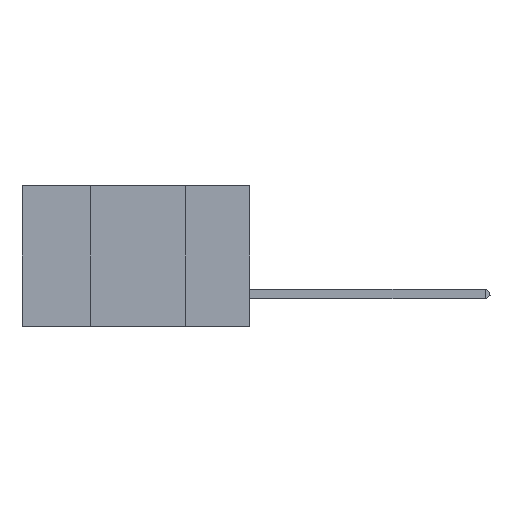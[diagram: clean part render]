
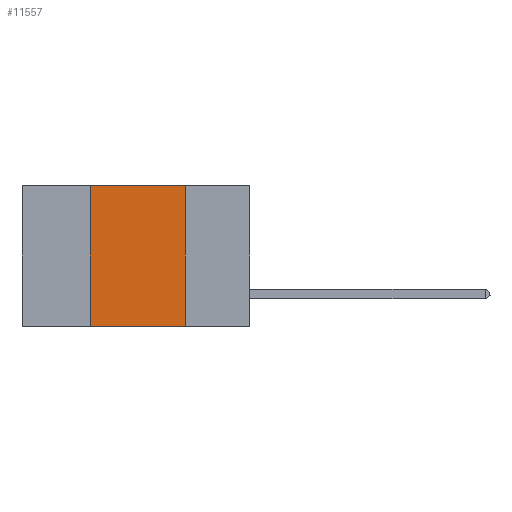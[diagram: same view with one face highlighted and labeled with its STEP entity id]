
A CAD part, left-side view. The second image highlights one B-rep face of the part: STEP entity #11557.
In plain terms, the highlighted planar face has unit normal (-1, 0, 0).
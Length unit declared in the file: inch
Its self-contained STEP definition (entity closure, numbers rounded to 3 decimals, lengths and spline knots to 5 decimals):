
#317 = VECTOR ( 'NONE', #8562, 39.37008 ) ;
#1373 = ORIENTED_EDGE ( 'NONE', *, *, #22876, .F. ) ;
#2792 = CARTESIAN_POINT ( 'NONE',  ( 0., 0.17, 0. ) ) ;
#3092 = PLANE ( 'NONE',  #29829 ) ;
#4129 = ORIENTED_EDGE ( 'NONE', *, *, #28291, .F. ) ;
#4709 = ORIENTED_EDGE ( 'NONE', *, *, #6818, .F. ) ;
#4942 = CARTESIAN_POINT ( 'NONE',  ( 0., 0.6, 0. ) ) ;
#5448 = DIRECTION ( 'NONE',  ( 0., -1., 0. ) ) ;
#5507 = VECTOR ( 'NONE', #21435, 39.37008 ) ;
#6730 = CARTESIAN_POINT ( 'NONE',  ( 0., 0.42, 0. ) ) ;
#6818 = EDGE_CURVE ( 'NONE', #15414, #7684, #13244, .T. ) ;
#7325 = EDGE_LOOP ( 'NONE', ( #1373, #4129, #4709, #10598 ) ) ;
#7684 = VERTEX_POINT ( 'NONE', #6730 ) ;
#7701 = VERTEX_POINT ( 'NONE', #27903 ) ;
#8562 = DIRECTION ( 'NONE',  ( 0., 0., 1. ) ) ;
#10029 = LINE ( 'NONE', #24080, #16336 ) ;
#10276 = DIRECTION ( 'NONE',  ( 0., -1., 0. ) ) ;
#10598 = ORIENTED_EDGE ( 'NONE', *, *, #15586, .T. ) ;
#10708 = CARTESIAN_POINT ( 'NONE',  ( 0., 0.42, 0. ) ) ;
#11557 = ADVANCED_FACE ( 'NONE', ( #23799 ), #3092, .F. ) ;
#13244 = LINE ( 'NONE', #10708, #317 ) ;
#15414 = VERTEX_POINT ( 'NONE', #24898 ) ;
#15586 = EDGE_CURVE ( 'NONE', #15414, #7701, #10029, .T. ) ;
#16336 = VECTOR ( 'NONE', #10276, 39.37008 ) ;
#17015 = DIRECTION ( 'NONE',  ( 1., 0., 0. ) ) ;
#18062 = LINE ( 'NONE', #25851, #5507 ) ;
#19432 = VECTOR ( 'NONE', #5448, 39.37008 ) ;
#19560 = CARTESIAN_POINT ( 'NONE',  ( 0., 0.6, 0. ) ) ;
#19880 = VERTEX_POINT ( 'NONE', #2792 ) ;
#21435 = DIRECTION ( 'NONE',  ( 0., 0., -1. ) ) ;
#22375 = LINE ( 'NONE', #4942, #19432 ) ;
#22876 = EDGE_CURVE ( 'NONE', #19880, #7701, #18062, .T. ) ;
#23799 = FACE_OUTER_BOUND ( 'NONE', #7325, .T. ) ;
#24080 = CARTESIAN_POINT ( 'NONE',  ( 0., 0.6, -0.37 ) ) ;
#24268 = DIRECTION ( 'NONE',  ( 0., 0., -1. ) ) ;
#24898 = CARTESIAN_POINT ( 'NONE',  ( 0., 0.42, -0.37 ) ) ;
#25851 = CARTESIAN_POINT ( 'NONE',  ( 0., 0.17, 0. ) ) ;
#27903 = CARTESIAN_POINT ( 'NONE',  ( 0., 0.17, -0.37 ) ) ;
#28291 = EDGE_CURVE ( 'NONE', #7684, #19880, #22375, .T. ) ;
#29829 = AXIS2_PLACEMENT_3D ( 'NONE', #19560, #17015, #24268 ) ;
